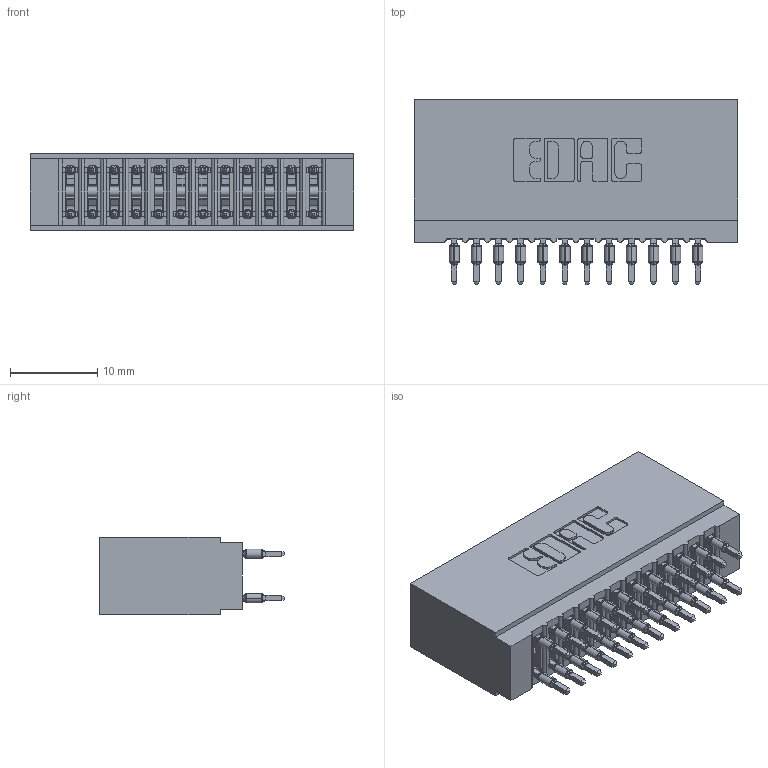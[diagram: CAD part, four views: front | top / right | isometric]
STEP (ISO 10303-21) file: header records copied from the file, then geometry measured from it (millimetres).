
FILE_DESCRIPTION (( 'STEP AP203' ), '1' );
FILE_NAME ('745-024-560-201.STEP', '2020-09-11T18:17:25', ( '' ), ( '' ), 'SwSTEP 2.0', 'SolidWorks 2020', '' );
FILE_SCHEMA (( 'CONFIG_CONTROL_DESIGN' ));
Length unit declared in the file: inch
Products named in the file (3): 745-292-001_560; 745-024-560-201; 745 Part_Insulator Option - 01
Assembly tree (25 placements, depth 2):
  745-024-560-201
    745 Part_Insulator Option - 01
    745-292-001_560  x24
Bounding box: 37.08 x 21.22 x 8.89 mm (x, y, z)
Volume: 3610.3 mm3; surface area: 7022.7 mm2
Topology: 25 solids, 25 shells, 2459 faces, 6726 edges, 4276 vertices
Faces by surface type: plane 1279, cylinder 556, bspline 480, torus 144
Entity records: 24627 total; most frequent: CARTESIAN_POINT 4785, ORIENTED_EDGE 4160, DIRECTION 3664, EDGE_CURVE 2080, VECTOR 1818, LINE 1818, VERTEX_POINT 1332, AXIS2_PLACEMENT_3D 923
